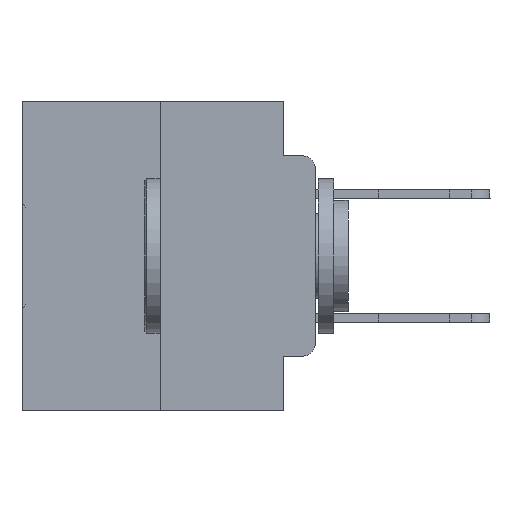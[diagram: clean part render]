
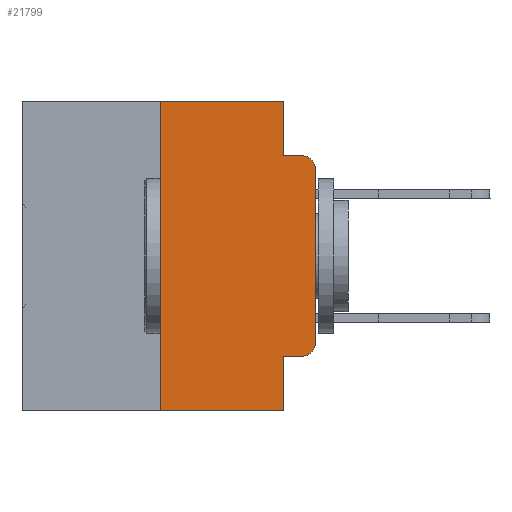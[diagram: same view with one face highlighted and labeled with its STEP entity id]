
A CAD part, left-side view. The second image highlights one B-rep face of the part: STEP entity #21799.
In plain terms, the highlighted planar face has unit normal (-1, 0, 0).
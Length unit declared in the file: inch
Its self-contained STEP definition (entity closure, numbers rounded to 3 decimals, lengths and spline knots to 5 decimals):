
#615 = LINE ( 'NONE', #32178, #17752 ) ;
#1235 = CARTESIAN_POINT ( 'NONE',  ( 0., 0., -0.3915 ) ) ;
#1692 = EDGE_CURVE ( 'NONE', #9961, #30604, #19749, .T. ) ;
#1868 = ORIENTED_EDGE ( 'NONE', *, *, #29404, .F. ) ;
#2170 = DIRECTION ( 'NONE',  ( 0., 0., -1. ) ) ;
#2756 = ORIENTED_EDGE ( 'NONE', *, *, #27772, .F. ) ;
#3683 = LINE ( 'NONE', #27288, #16439 ) ;
#4918 = CARTESIAN_POINT ( 'NONE',  ( 0., 0.473, 0. ) ) ;
#5697 = VERTEX_POINT ( 'NONE', #17595 ) ;
#5754 = VERTEX_POINT ( 'NONE', #25300 ) ;
#6444 = ORIENTED_EDGE ( 'NONE', *, *, #1692, .T. ) ;
#6816 = DIRECTION ( 'NONE',  ( -1., 0., 0. ) ) ;
#7016 = DIRECTION ( 'NONE',  ( 0., -1., 0. ) ) ;
#7483 = DIRECTION ( 'NONE',  ( 0., 0., -1. ) ) ;
#7498 = LINE ( 'NONE', #22199, #27689 ) ;
#8478 = LINE ( 'NONE', #13064, #14486 ) ;
#9140 = ORIENTED_EDGE ( 'NONE', *, *, #19576, .F. ) ;
#9721 = ORIENTED_EDGE ( 'NONE', *, *, #10881, .T. ) ;
#9961 = VERTEX_POINT ( 'NONE', #1235 ) ;
#10085 = ORIENTED_EDGE ( 'NONE', *, *, #26550, .T. ) ;
#10195 = CARTESIAN_POINT ( 'NONE',  ( 0., 0.02, -0.4115 ) ) ;
#10881 = EDGE_CURVE ( 'NONE', #10970, #9961, #17066, .T. ) ;
#10970 = VERTEX_POINT ( 'NONE', #10195 ) ;
#11164 = VECTOR ( 'NONE', #2170, 39.37008 ) ;
#11505 = AXIS2_PLACEMENT_3D ( 'NONE', #22003, #6816, #24572 ) ;
#12175 = DIRECTION ( 'NONE',  ( 0., 0., 1. ) ) ;
#12418 = CARTESIAN_POINT ( 'NONE',  ( 0., 0.02, -0.3915 ) ) ;
#13036 = VECTOR ( 'NONE', #24387, 39.37008 ) ;
#13064 = CARTESIAN_POINT ( 'NONE',  ( 0., 0.051, -0.4115 ) ) ;
#13694 = ORIENTED_EDGE ( 'NONE', *, *, #14282, .T. ) ;
#14282 = EDGE_CURVE ( 'NONE', #5754, #10970, #8478, .T. ) ;
#14354 = CARTESIAN_POINT ( 'NONE',  ( 0., 0.051, 0. ) ) ;
#14486 = VECTOR ( 'NONE', #15621, 39.37008 ) ;
#14975 = DIRECTION ( 'NONE',  ( 0., 0., -1. ) ) ;
#15466 = VERTEX_POINT ( 'NONE', #18091 ) ;
#15621 = DIRECTION ( 'NONE',  ( 0., -1., 0. ) ) ;
#16439 = VECTOR ( 'NONE', #12175, 39.37008 ) ;
#16467 = CARTESIAN_POINT ( 'NONE',  ( 0., 0.051, -0.5 ) ) ;
#16637 = DIRECTION ( 'NONE',  ( 0., -1., 0. ) ) ;
#17066 = CIRCLE ( 'NONE', #22461, 0.02 ) ;
#17224 = DIRECTION ( 'NONE',  ( 0., -1., 0. ) ) ;
#17525 = PLANE ( 'NONE',  #27973 ) ;
#17595 = CARTESIAN_POINT ( 'NONE',  ( 0., 0.25, 0. ) ) ;
#17752 = VECTOR ( 'NONE', #17224, 39.37008 ) ;
#17795 = CARTESIAN_POINT ( 'NONE',  ( 0., 0.051, -0.0885 ) ) ;
#17911 = LINE ( 'NONE', #32267, #11164 ) ;
#18091 = CARTESIAN_POINT ( 'NONE',  ( 0., 0.02, -0.0885 ) ) ;
#18557 = FACE_OUTER_BOUND ( 'NONE', #21490, .T. ) ;
#19336 = EDGE_CURVE ( 'NONE', #5754, #22751, #26218, .T. ) ;
#19485 = VECTOR ( 'NONE', #28059, 39.37008 ) ;
#19576 = EDGE_CURVE ( 'NONE', #5697, #22862, #25806, .T. ) ;
#19749 = LINE ( 'NONE', #28531, #13036 ) ;
#20731 = CIRCLE ( 'NONE', #11505, 0.02 ) ;
#21490 = EDGE_LOOP ( 'NONE', ( #6444, #21546, #1868, #2756, #9140, #27070, #10085, #28237, #13694, #9721 ) ) ;
#21546 = ORIENTED_EDGE ( 'NONE', *, *, #32607, .T. ) ;
#21799 = ADVANCED_FACE ( 'NONE', ( #18557 ), #17525, .F. ) ;
#22003 = CARTESIAN_POINT ( 'NONE',  ( 0., 0.02, -0.1085 ) ) ;
#22199 = CARTESIAN_POINT ( 'NONE',  ( 0., 0.473, -0.5 ) ) ;
#22461 = AXIS2_PLACEMENT_3D ( 'NONE', #12418, #29956, #14975 ) ;
#22658 = DIRECTION ( 'NONE',  ( 1., 0., 0. ) ) ;
#22751 = VERTEX_POINT ( 'NONE', #16467 ) ;
#22862 = VERTEX_POINT ( 'NONE', #14354 ) ;
#24387 = DIRECTION ( 'NONE',  ( 0., 0., 1. ) ) ;
#24424 = EDGE_CURVE ( 'NONE', #30218, #5697, #3683, .T. ) ;
#24572 = DIRECTION ( 'NONE',  ( 0., 0., -1. ) ) ;
#25300 = CARTESIAN_POINT ( 'NONE',  ( 0., 0.051, -0.4115 ) ) ;
#25806 = LINE ( 'NONE', #31512, #26594 ) ;
#26218 = LINE ( 'NONE', #30478, #19485 ) ;
#26550 = EDGE_CURVE ( 'NONE', #30218, #22751, #7498, .T. ) ;
#26594 = VECTOR ( 'NONE', #16637, 39.37008 ) ;
#27047 = CARTESIAN_POINT ( 'NONE',  ( 0., 0., -0.1085 ) ) ;
#27070 = ORIENTED_EDGE ( 'NONE', *, *, #24424, .F. ) ;
#27288 = CARTESIAN_POINT ( 'NONE',  ( 0., 0.25, 0. ) ) ;
#27689 = VECTOR ( 'NONE', #7016, 39.37008 ) ;
#27772 = EDGE_CURVE ( 'NONE', #22862, #28917, #17911, .T. ) ;
#27973 = AXIS2_PLACEMENT_3D ( 'NONE', #4918, #22658, #7483 ) ;
#28059 = DIRECTION ( 'NONE',  ( 0., 0., -1. ) ) ;
#28237 = ORIENTED_EDGE ( 'NONE', *, *, #19336, .F. ) ;
#28531 = CARTESIAN_POINT ( 'NONE',  ( 0., 0., 0. ) ) ;
#28917 = VERTEX_POINT ( 'NONE', #17795 ) ;
#29404 = EDGE_CURVE ( 'NONE', #28917, #15466, #615, .T. ) ;
#29956 = DIRECTION ( 'NONE',  ( -1., 0., 0. ) ) ;
#30218 = VERTEX_POINT ( 'NONE', #30554 ) ;
#30478 = CARTESIAN_POINT ( 'NONE',  ( 0., 0.051, 0. ) ) ;
#30554 = CARTESIAN_POINT ( 'NONE',  ( 0., 0.25, -0.5 ) ) ;
#30604 = VERTEX_POINT ( 'NONE', #27047 ) ;
#31512 = CARTESIAN_POINT ( 'NONE',  ( 0., 0.473, 0. ) ) ;
#32178 = CARTESIAN_POINT ( 'NONE',  ( 0., 0.051, -0.0885 ) ) ;
#32267 = CARTESIAN_POINT ( 'NONE',  ( 0., 0.051, 0. ) ) ;
#32607 = EDGE_CURVE ( 'NONE', #30604, #15466, #20731, .T. ) ;
